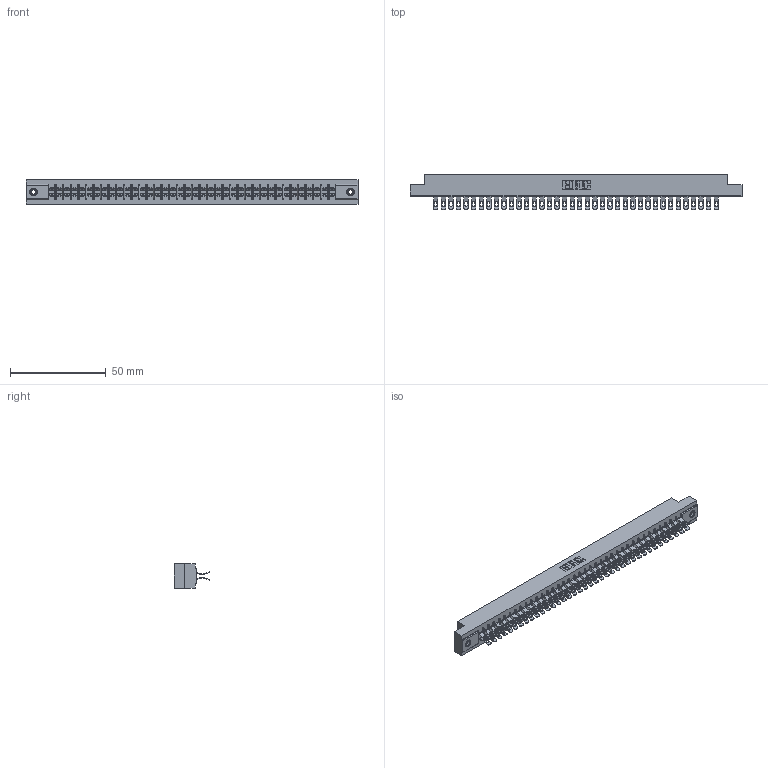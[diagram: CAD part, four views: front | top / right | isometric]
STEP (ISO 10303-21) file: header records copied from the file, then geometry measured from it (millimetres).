
FILE_DESCRIPTION (( 'STEP AP203' ), '1' );
FILE_NAME ('355-076-555-208.STEP', '2019-09-13T13:25:04', ( '' ), ( '' ), 'SwSTEP 2.0', 'SolidWorks 2016', '' );
FILE_SCHEMA (( 'CONFIG_CONTROL_DESIGN' ));
Length unit declared in the file: inch
Products named in the file (4): 355-076-555-208; 345-250-001_345-250-003-102; 305 Part_.156 Dia; 305-290-001_555
Assembly tree (79 placements, depth 2):
  355-076-555-208
    305 Part_.156 Dia
    305-290-001_555  x76
    345-250-001_345-250-003-102  x2
Bounding box: 173.58 x 18.41 x 12.7 mm (x, y, z)
Volume: 18296.9 mm3; surface area: 24650.1 mm2
Topology: 79 solids, 79 shells, 5192 faces, 15462 edges, 10096 vertices
Faces by surface type: plane 2532, cylinder 2492, sphere 152, cone 12, torus 4
Entity records: 43440 total; most frequent: CARTESIAN_POINT 7189, ORIENTED_EDGE 7120, DIRECTION 6962, EDGE_CURVE 3560, LINE 2852, VECTOR 2852, VERTEX_POINT 2266, AXIS2_PLACEMENT_3D 2055
